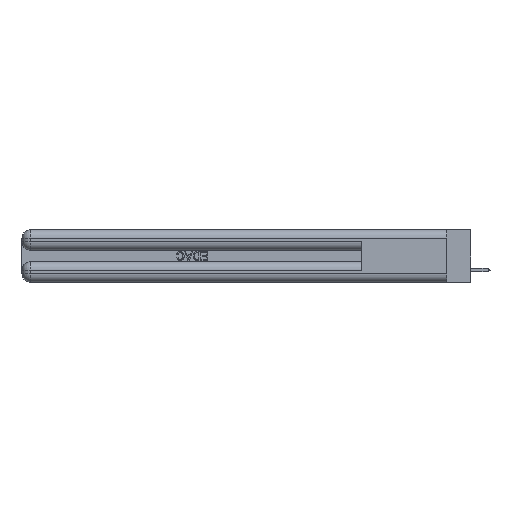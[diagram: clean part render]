
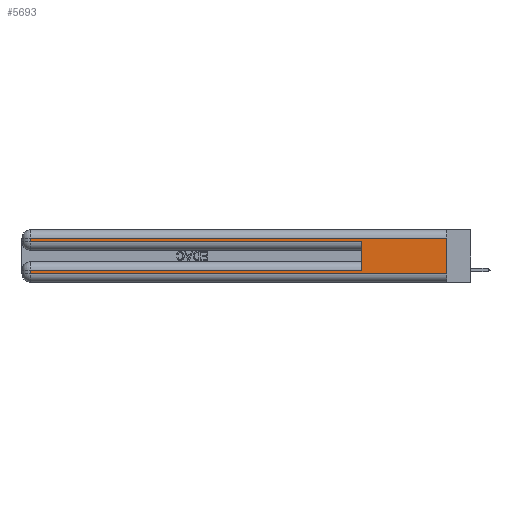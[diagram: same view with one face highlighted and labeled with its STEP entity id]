
A CAD part, left-side view. The second image highlights one B-rep face of the part: STEP entity #5693.
In plain terms, the highlighted planar face has unit normal (-1, 0, 0).
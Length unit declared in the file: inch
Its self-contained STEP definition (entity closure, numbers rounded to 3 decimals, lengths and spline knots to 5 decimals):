
#232 = LINE ( 'NONE', #41223, #33075 ) ;
#1734 = CARTESIAN_POINT ( 'NONE',  ( 0., 0., 0.31 ) ) ;
#1762 = CARTESIAN_POINT ( 'NONE',  ( 0., 2.94, 0.085 ) ) ;
#2151 = VECTOR ( 'NONE', #2414, 39.37008 ) ;
#2414 = DIRECTION ( 'NONE',  ( 0., 0., 1. ) ) ;
#2450 = ORIENTED_EDGE ( 'NONE', *, *, #9966, .T. ) ;
#2536 = CARTESIAN_POINT ( 'NONE',  ( 0., 2.94, 0.31 ) ) ;
#3243 = LINE ( 'NONE', #26581, #14416 ) ;
#3375 = EDGE_CURVE ( 'NONE', #23664, #5074, #5431, .T. ) ;
#4239 = EDGE_CURVE ( 'NONE', #23510, #35087, #12888, .T. ) ;
#5074 = VERTEX_POINT ( 'NONE', #24539 ) ;
#5120 = DIRECTION ( 'NONE',  ( 0., -1., 0. ) ) ;
#5297 = LINE ( 'NONE', #21082, #38122 ) ;
#5431 = LINE ( 'NONE', #9584, #12051 ) ;
#5453 = PLANE ( 'NONE',  #39923 ) ;
#5693 = ADVANCED_FACE ( 'NONE', ( #28197 ), #5453, .F. ) ;
#5941 = VECTOR ( 'NONE', #6302, 39.37008 ) ;
#6302 = DIRECTION ( 'NONE',  ( 0., 1., 0. ) ) ;
#7624 = CARTESIAN_POINT ( 'NONE',  ( 0., 0.6, 0.285 ) ) ;
#8286 = ORIENTED_EDGE ( 'NONE', *, *, #4239, .F. ) ;
#9584 = CARTESIAN_POINT ( 'NONE',  ( 0., 2.94, 0.37 ) ) ;
#9700 = CARTESIAN_POINT ( 'NONE',  ( 0., 0., 0.085 ) ) ;
#9966 = EDGE_CURVE ( 'NONE', #31924, #35087, #5297, .T. ) ;
#10607 = ORIENTED_EDGE ( 'NONE', *, *, #11845, .T. ) ;
#11165 = CARTESIAN_POINT ( 'NONE',  ( 0., 2.94, 0.37 ) ) ;
#11314 = ORIENTED_EDGE ( 'NONE', *, *, #28464, .T. ) ;
#11527 = DIRECTION ( 'NONE',  ( 0., 0., -1. ) ) ;
#11845 = EDGE_CURVE ( 'NONE', #33029, #31924, #16714, .T. ) ;
#12051 = VECTOR ( 'NONE', #37168, 39.37008 ) ;
#12888 = LINE ( 'NONE', #38386, #2151 ) ;
#13492 = DIRECTION ( 'NONE',  ( 0., -1., 0. ) ) ;
#14416 = VECTOR ( 'NONE', #13492, 39.37008 ) ;
#14435 = CARTESIAN_POINT ( 'NONE',  ( 0., 0., 0.06 ) ) ;
#15915 = LINE ( 'NONE', #18457, #18488 ) ;
#16165 = EDGE_CURVE ( 'NONE', #24222, #17203, #15915, .T. ) ;
#16714 = LINE ( 'NONE', #11165, #41906 ) ;
#17203 = VERTEX_POINT ( 'NONE', #14435 ) ;
#18002 = DIRECTION ( 'NONE',  ( 0., 0., -1. ) ) ;
#18457 = CARTESIAN_POINT ( 'NONE',  ( 0., 0., 0.37 ) ) ;
#18488 = VECTOR ( 'NONE', #11527, 39.37008 ) ;
#19076 = CARTESIAN_POINT ( 'NONE',  ( 0., 2.94, 0.285 ) ) ;
#21082 = CARTESIAN_POINT ( 'NONE',  ( 0., 0., 0.285 ) ) ;
#21105 = DIRECTION ( 'NONE',  ( 1., 0., 0. ) ) ;
#22534 = EDGE_LOOP ( 'NONE', ( #36877, #27858, #10607, #2450, #8286, #27346, #33827, #11314 ) ) ;
#23510 = VERTEX_POINT ( 'NONE', #32807 ) ;
#23664 = VERTEX_POINT ( 'NONE', #1762 ) ;
#24222 = VERTEX_POINT ( 'NONE', #1734 ) ;
#24539 = CARTESIAN_POINT ( 'NONE',  ( 0., 2.94, 0.06 ) ) ;
#25644 = CARTESIAN_POINT ( 'NONE',  ( 0., 0., 0.37 ) ) ;
#26578 = EDGE_CURVE ( 'NONE', #24222, #33029, #232, .T. ) ;
#26581 = CARTESIAN_POINT ( 'NONE',  ( 0., 0., 0.06 ) ) ;
#27346 = ORIENTED_EDGE ( 'NONE', *, *, #30667, .T. ) ;
#27858 = ORIENTED_EDGE ( 'NONE', *, *, #26578, .T. ) ;
#28197 = FACE_OUTER_BOUND ( 'NONE', #22534, .T. ) ;
#28464 = EDGE_CURVE ( 'NONE', #5074, #17203, #3243, .T. ) ;
#30667 = EDGE_CURVE ( 'NONE', #23510, #23664, #32075, .T. ) ;
#31924 = VERTEX_POINT ( 'NONE', #19076 ) ;
#32075 = LINE ( 'NONE', #9700, #5941 ) ;
#32807 = CARTESIAN_POINT ( 'NONE',  ( 0., 0.6, 0.085 ) ) ;
#33029 = VERTEX_POINT ( 'NONE', #2536 ) ;
#33075 = VECTOR ( 'NONE', #34786, 39.37008 ) ;
#33827 = ORIENTED_EDGE ( 'NONE', *, *, #3375, .T. ) ;
#34786 = DIRECTION ( 'NONE',  ( 0., 1., 0. ) ) ;
#35087 = VERTEX_POINT ( 'NONE', #7624 ) ;
#36877 = ORIENTED_EDGE ( 'NONE', *, *, #16165, .F. ) ;
#37168 = DIRECTION ( 'NONE',  ( 0., 0., -1. ) ) ;
#38122 = VECTOR ( 'NONE', #5120, 39.37008 ) ;
#38386 = CARTESIAN_POINT ( 'NONE',  ( 0., 0.6, 0.145 ) ) ;
#39923 = AXIS2_PLACEMENT_3D ( 'NONE', #25644, #21105, #18002 ) ;
#40543 = DIRECTION ( 'NONE',  ( 0., 0., -1. ) ) ;
#41223 = CARTESIAN_POINT ( 'NONE',  ( 0., 0., 0.31 ) ) ;
#41906 = VECTOR ( 'NONE', #40543, 39.37008 ) ;
